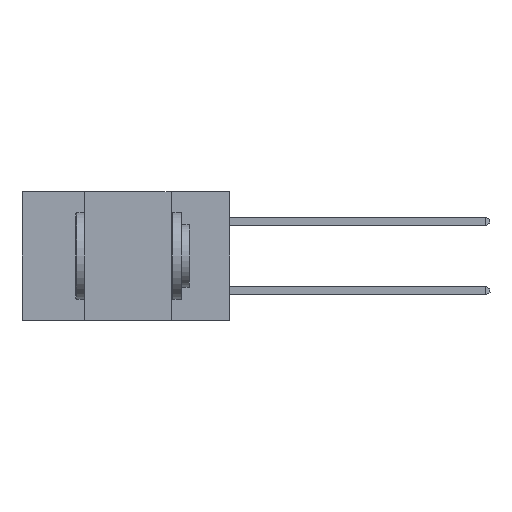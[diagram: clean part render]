
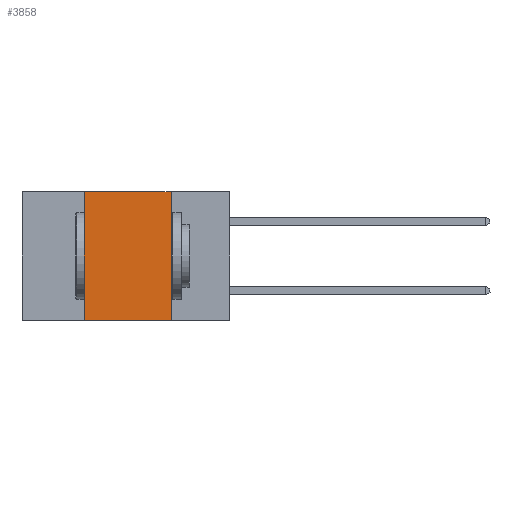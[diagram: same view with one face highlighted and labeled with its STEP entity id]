
A CAD part, left-side view. The second image highlights one B-rep face of the part: STEP entity #3858.
In plain terms, the highlighted planar face has unit normal (-1, 0, 0).
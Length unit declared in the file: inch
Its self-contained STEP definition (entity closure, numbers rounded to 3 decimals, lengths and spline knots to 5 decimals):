
#289 = FACE_OUTER_BOUND ( 'NONE', #6875, .T. ) ;
#537 = CARTESIAN_POINT ( 'NONE',  ( 0., 0.42, 0. ) ) ;
#689 = VECTOR ( 'NONE', #2659, 39.37008 ) ;
#1108 = VECTOR ( 'NONE', #2315, 39.37008 ) ;
#1707 = ORIENTED_EDGE ( 'NONE', *, *, #3768, .F. ) ;
#2315 = DIRECTION ( 'NONE',  ( 0., -1., 0. ) ) ;
#2659 = DIRECTION ( 'NONE',  ( 0., -1., 0. ) ) ;
#2683 = CARTESIAN_POINT ( 'NONE',  ( 0., 0.6, 0. ) ) ;
#2743 = ORIENTED_EDGE ( 'NONE', *, *, #10292, .F. ) ;
#2884 = LINE ( 'NONE', #4100, #1108 ) ;
#3080 = AXIS2_PLACEMENT_3D ( 'NONE', #2683, #9740, #6247 ) ;
#3545 = VERTEX_POINT ( 'NONE', #3951 ) ;
#3700 = CARTESIAN_POINT ( 'NONE',  ( 0., 0.17, 0. ) ) ;
#3768 = EDGE_CURVE ( 'NONE', #8175, #6008, #2884, .T. ) ;
#3858 = ADVANCED_FACE ( 'NONE', ( #289 ), #8824, .F. ) ;
#3951 = CARTESIAN_POINT ( 'NONE',  ( 0., 0.42, -0.37 ) ) ;
#3972 = LINE ( 'NONE', #3700, #7565 ) ;
#4100 = CARTESIAN_POINT ( 'NONE',  ( 0., 0.6, 0. ) ) ;
#4352 = EDGE_CURVE ( 'NONE', #3545, #5300, #6579, .T. ) ;
#4584 = DIRECTION ( 'NONE',  ( 0., 0., -1. ) ) ;
#5237 = CARTESIAN_POINT ( 'NONE',  ( 0., 0.6, -0.37 ) ) ;
#5300 = VERTEX_POINT ( 'NONE', #10330 ) ;
#5976 = CARTESIAN_POINT ( 'NONE',  ( 0., 0.17, 0. ) ) ;
#6008 = VERTEX_POINT ( 'NONE', #5976 ) ;
#6247 = DIRECTION ( 'NONE',  ( 0., 0., -1. ) ) ;
#6579 = LINE ( 'NONE', #5237, #689 ) ;
#6871 = VECTOR ( 'NONE', #8491, 39.37008 ) ;
#6875 = EDGE_LOOP ( 'NONE', ( #8735, #1707, #2743, #11106 ) ) ;
#7565 = VECTOR ( 'NONE', #4584, 39.37008 ) ;
#7706 = CARTESIAN_POINT ( 'NONE',  ( 0., 0.42, 0. ) ) ;
#8175 = VERTEX_POINT ( 'NONE', #7706 ) ;
#8394 = LINE ( 'NONE', #537, #6871 ) ;
#8491 = DIRECTION ( 'NONE',  ( 0., 0., 1. ) ) ;
#8735 = ORIENTED_EDGE ( 'NONE', *, *, #8826, .F. ) ;
#8824 = PLANE ( 'NONE',  #3080 ) ;
#8826 = EDGE_CURVE ( 'NONE', #6008, #5300, #3972, .T. ) ;
#9740 = DIRECTION ( 'NONE',  ( 1., 0., 0. ) ) ;
#10292 = EDGE_CURVE ( 'NONE', #3545, #8175, #8394, .T. ) ;
#10330 = CARTESIAN_POINT ( 'NONE',  ( 0., 0.17, -0.37 ) ) ;
#11106 = ORIENTED_EDGE ( 'NONE', *, *, #4352, .T. ) ;
